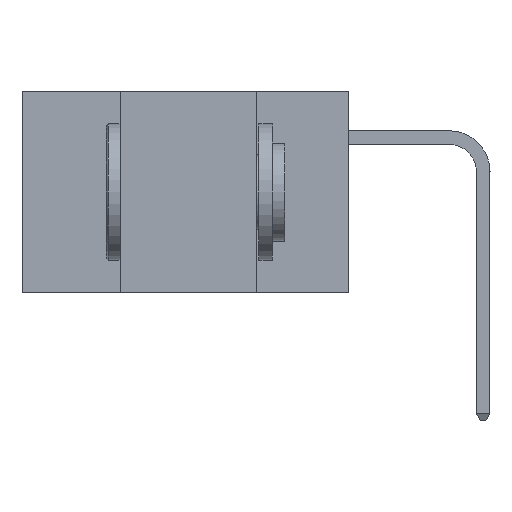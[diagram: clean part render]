
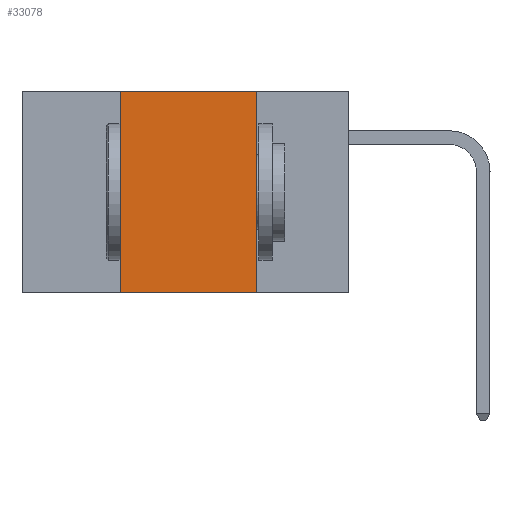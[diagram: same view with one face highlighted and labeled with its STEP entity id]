
A CAD part, left-side view. The second image highlights one B-rep face of the part: STEP entity #33078.
In plain terms, the highlighted planar face has unit normal (-1, 0, 0).
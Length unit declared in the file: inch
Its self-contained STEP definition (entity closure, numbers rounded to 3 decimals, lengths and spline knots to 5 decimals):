
#526 = DIRECTION ( 'NONE',  ( 0., 0., 1. ) ) ;
#2182 = DIRECTION ( 'NONE',  ( 1., 0., 0. ) ) ;
#3340 = ORIENTED_EDGE ( 'NONE', *, *, #21011, .T. ) ;
#3690 = EDGE_CURVE ( 'NONE', #35571, #13251, #9460, .T. ) ;
#4577 = EDGE_LOOP ( 'NONE', ( #9545, #24393, #17800, #3340 ) ) ;
#4783 = CARTESIAN_POINT ( 'NONE',  ( 0., 0.6, 0. ) ) ;
#7050 = DIRECTION ( 'NONE',  ( 0., -1., 0. ) ) ;
#7467 = EDGE_CURVE ( 'NONE', #30127, #35571, #26794, .T. ) ;
#7604 = CARTESIAN_POINT ( 'NONE',  ( 0., 0.17, 0. ) ) ;
#7726 = DIRECTION ( 'NONE',  ( 0., 0., -1. ) ) ;
#7735 = DIRECTION ( 'NONE',  ( 0., -1., 0. ) ) ;
#8768 = CARTESIAN_POINT ( 'NONE',  ( 0., 0.17, 0. ) ) ;
#9460 = LINE ( 'NONE', #7604, #31597 ) ;
#9545 = ORIENTED_EDGE ( 'NONE', *, *, #3690, .F. ) ;
#9807 = VERTEX_POINT ( 'NONE', #29166 ) ;
#13251 = VERTEX_POINT ( 'NONE', #21219 ) ;
#14350 = VECTOR ( 'NONE', #526, 39.37008 ) ;
#15663 = CARTESIAN_POINT ( 'NONE',  ( 0., 0.6, -0.37 ) ) ;
#15738 = VECTOR ( 'NONE', #7050, 39.37008 ) ;
#16393 = VECTOR ( 'NONE', #7735, 39.37008 ) ;
#17800 = ORIENTED_EDGE ( 'NONE', *, *, #31536, .F. ) ;
#20812 = CARTESIAN_POINT ( 'NONE',  ( 0., 0.42, 0. ) ) ;
#21011 = EDGE_CURVE ( 'NONE', #9807, #13251, #23456, .T. ) ;
#21219 = CARTESIAN_POINT ( 'NONE',  ( 0., 0.17, -0.37 ) ) ;
#22458 = DIRECTION ( 'NONE',  ( 0., 0., -1. ) ) ;
#23456 = LINE ( 'NONE', #15663, #15738 ) ;
#24393 = ORIENTED_EDGE ( 'NONE', *, *, #7467, .F. ) ;
#24404 = FACE_OUTER_BOUND ( 'NONE', #4577, .T. ) ;
#24535 = AXIS2_PLACEMENT_3D ( 'NONE', #25227, #2182, #22458 ) ;
#25227 = CARTESIAN_POINT ( 'NONE',  ( 0., 0.6, 0. ) ) ;
#26794 = LINE ( 'NONE', #4783, #16393 ) ;
#29166 = CARTESIAN_POINT ( 'NONE',  ( 0., 0.42, -0.37 ) ) ;
#29720 = LINE ( 'NONE', #20812, #14350 ) ;
#30127 = VERTEX_POINT ( 'NONE', #37120 ) ;
#31020 = PLANE ( 'NONE',  #24535 ) ;
#31536 = EDGE_CURVE ( 'NONE', #9807, #30127, #29720, .T. ) ;
#31597 = VECTOR ( 'NONE', #7726, 39.37008 ) ;
#33078 = ADVANCED_FACE ( 'NONE', ( #24404 ), #31020, .F. ) ;
#35571 = VERTEX_POINT ( 'NONE', #8768 ) ;
#37120 = CARTESIAN_POINT ( 'NONE',  ( 0., 0.42, 0. ) ) ;
